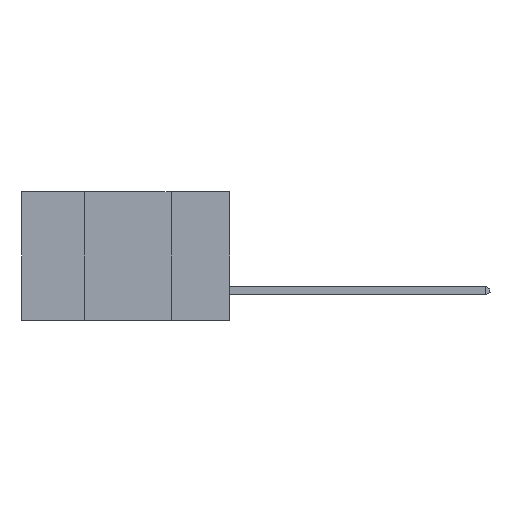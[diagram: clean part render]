
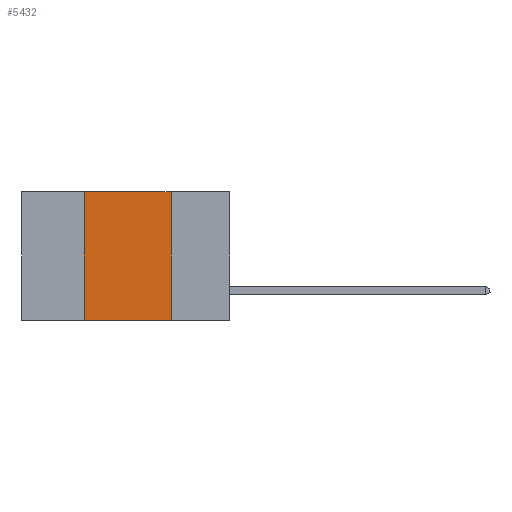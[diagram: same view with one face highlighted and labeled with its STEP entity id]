
A CAD part, left-side view. The second image highlights one B-rep face of the part: STEP entity #5432.
In plain terms, the highlighted planar face has unit normal (-1, 0, 0).
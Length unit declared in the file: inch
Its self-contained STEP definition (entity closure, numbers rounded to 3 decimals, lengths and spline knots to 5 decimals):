
#255 = DIRECTION ( 'NONE',  ( 0., -1., 0. ) ) ;
#438 = LINE ( 'NONE', #6109, #16588 ) ;
#1427 = AXIS2_PLACEMENT_3D ( 'NONE', #11136, #16869, #2901 ) ;
#2901 = DIRECTION ( 'NONE',  ( 0., 0., -1. ) ) ;
#4417 = CARTESIAN_POINT ( 'NONE',  ( 0., 0.6, 0. ) ) ;
#4521 = CARTESIAN_POINT ( 'NONE',  ( 0., 0.17, 0. ) ) ;
#4768 = EDGE_CURVE ( 'NONE', #13826, #5898, #13219, .T. ) ;
#4960 = ORIENTED_EDGE ( 'NONE', *, *, #11432, .F. ) ;
#5432 = ADVANCED_FACE ( 'NONE', ( #10185 ), #15488, .F. ) ;
#5898 = VERTEX_POINT ( 'NONE', #11892 ) ;
#5936 = DIRECTION ( 'NONE',  ( 0., 0., -1. ) ) ;
#6094 = VERTEX_POINT ( 'NONE', #16594 ) ;
#6109 = CARTESIAN_POINT ( 'NONE',  ( 0., 0.42, 0. ) ) ;
#6623 = EDGE_CURVE ( 'NONE', #6094, #13631, #438, .T. ) ;
#7302 = CARTESIAN_POINT ( 'NONE',  ( 0., 0.17, 0. ) ) ;
#7508 = DIRECTION ( 'NONE',  ( 0., -1., 0. ) ) ;
#9219 = LINE ( 'NONE', #4417, #14575 ) ;
#9568 = ORIENTED_EDGE ( 'NONE', *, *, #9611, .T. ) ;
#9611 = EDGE_CURVE ( 'NONE', #6094, #5898, #11186, .T. ) ;
#9950 = EDGE_LOOP ( 'NONE', ( #11460, #4960, #15057, #9568 ) ) ;
#10185 = FACE_OUTER_BOUND ( 'NONE', #9950, .T. ) ;
#11136 = CARTESIAN_POINT ( 'NONE',  ( 0., 0.6, 0. ) ) ;
#11186 = LINE ( 'NONE', #12869, #14447 ) ;
#11432 = EDGE_CURVE ( 'NONE', #13631, #13826, #9219, .T. ) ;
#11460 = ORIENTED_EDGE ( 'NONE', *, *, #4768, .F. ) ;
#11892 = CARTESIAN_POINT ( 'NONE',  ( 0., 0.17, -0.37 ) ) ;
#12869 = CARTESIAN_POINT ( 'NONE',  ( 0., 0.6, -0.37 ) ) ;
#13219 = LINE ( 'NONE', #4521, #15157 ) ;
#13631 = VERTEX_POINT ( 'NONE', #16097 ) ;
#13826 = VERTEX_POINT ( 'NONE', #7302 ) ;
#14447 = VECTOR ( 'NONE', #7508, 39.37008 ) ;
#14575 = VECTOR ( 'NONE', #255, 39.37008 ) ;
#15057 = ORIENTED_EDGE ( 'NONE', *, *, #6623, .F. ) ;
#15157 = VECTOR ( 'NONE', #5936, 39.37008 ) ;
#15488 = PLANE ( 'NONE',  #1427 ) ;
#15795 = DIRECTION ( 'NONE',  ( 0., 0., 1. ) ) ;
#16097 = CARTESIAN_POINT ( 'NONE',  ( 0., 0.42, 0. ) ) ;
#16588 = VECTOR ( 'NONE', #15795, 39.37008 ) ;
#16594 = CARTESIAN_POINT ( 'NONE',  ( 0., 0.42, -0.37 ) ) ;
#16869 = DIRECTION ( 'NONE',  ( 1., 0., 0. ) ) ;
